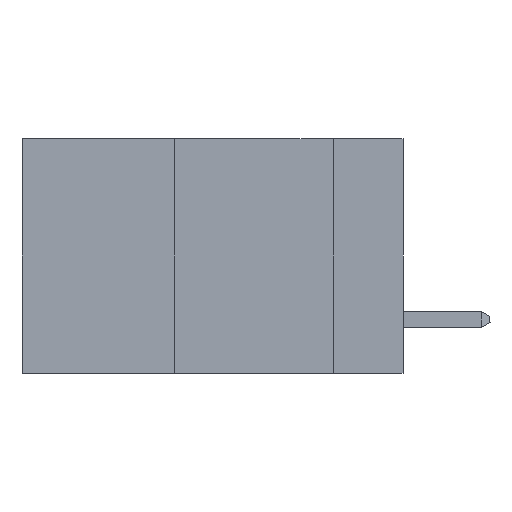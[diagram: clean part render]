
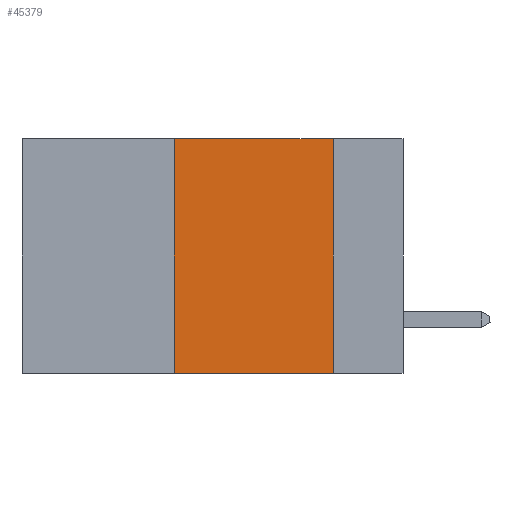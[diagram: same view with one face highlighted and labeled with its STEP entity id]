
A CAD part, left-side view. The second image highlights one B-rep face of the part: STEP entity #45379.
In plain terms, the highlighted planar face has unit normal (-1, 0, 0).
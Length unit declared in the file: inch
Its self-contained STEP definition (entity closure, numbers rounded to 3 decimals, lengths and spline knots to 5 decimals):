
#455 = DIRECTION ( 'NONE',  ( 1., 0., 0. ) ) ;
#952 = EDGE_CURVE ( 'NONE', #37349, #40477, #7861, .T. ) ;
#1590 = FACE_OUTER_BOUND ( 'NONE', #9610, .T. ) ;
#4086 = VECTOR ( 'NONE', #19787, 39.37008 ) ;
#5461 = LINE ( 'NONE', #32705, #21979 ) ;
#5653 = ORIENTED_EDGE ( 'NONE', *, *, #952, .F. ) ;
#7397 = AXIS2_PLACEMENT_3D ( 'NONE', #18576, #455, #44362 ) ;
#7861 = LINE ( 'NONE', #26657, #14749 ) ;
#9610 = EDGE_LOOP ( 'NONE', ( #5653, #25426, #14672, #46212 ) ) ;
#11093 = VERTEX_POINT ( 'NONE', #18035 ) ;
#14000 = CARTESIAN_POINT ( 'NONE',  ( 0., 0.6, 0. ) ) ;
#14672 = ORIENTED_EDGE ( 'NONE', *, *, #29312, .F. ) ;
#14749 = VECTOR ( 'NONE', #33986, 39.37008 ) ;
#18035 = CARTESIAN_POINT ( 'NONE',  ( 0., 0.36, 0. ) ) ;
#18576 = CARTESIAN_POINT ( 'NONE',  ( 0., 0.6, 0. ) ) ;
#19787 = DIRECTION ( 'NONE',  ( 0., -1., 0. ) ) ;
#21250 = DIRECTION ( 'NONE',  ( 0., -1., 0. ) ) ;
#21979 = VECTOR ( 'NONE', #32375, 39.37008 ) ;
#22209 = LINE ( 'NONE', #30484, #4086 ) ;
#22536 = PLANE ( 'NONE',  #7397 ) ;
#23446 = CARTESIAN_POINT ( 'NONE',  ( 0., 0.11, -0.37 ) ) ;
#24925 = LINE ( 'NONE', #14000, #36856 ) ;
#25426 = ORIENTED_EDGE ( 'NONE', *, *, #36216, .F. ) ;
#26657 = CARTESIAN_POINT ( 'NONE',  ( 0., 0.11, 0. ) ) ;
#29312 = EDGE_CURVE ( 'NONE', #34392, #11093, #5461, .T. ) ;
#29938 = CARTESIAN_POINT ( 'NONE',  ( 0., 0.11, 0. ) ) ;
#30484 = CARTESIAN_POINT ( 'NONE',  ( 0., 0.6, -0.37 ) ) ;
#32375 = DIRECTION ( 'NONE',  ( 0., 0., 1. ) ) ;
#32705 = CARTESIAN_POINT ( 'NONE',  ( 0., 0.36, 0. ) ) ;
#33986 = DIRECTION ( 'NONE',  ( 0., 0., -1. ) ) ;
#34392 = VERTEX_POINT ( 'NONE', #43079 ) ;
#34702 = EDGE_CURVE ( 'NONE', #34392, #40477, #22209, .T. ) ;
#36216 = EDGE_CURVE ( 'NONE', #11093, #37349, #24925, .T. ) ;
#36856 = VECTOR ( 'NONE', #21250, 39.37008 ) ;
#37349 = VERTEX_POINT ( 'NONE', #29938 ) ;
#40477 = VERTEX_POINT ( 'NONE', #23446 ) ;
#43079 = CARTESIAN_POINT ( 'NONE',  ( 0., 0.36, -0.37 ) ) ;
#44362 = DIRECTION ( 'NONE',  ( 0., 0., -1. ) ) ;
#45379 = ADVANCED_FACE ( 'NONE', ( #1590 ), #22536, .F. ) ;
#46212 = ORIENTED_EDGE ( 'NONE', *, *, #34702, .T. ) ;
